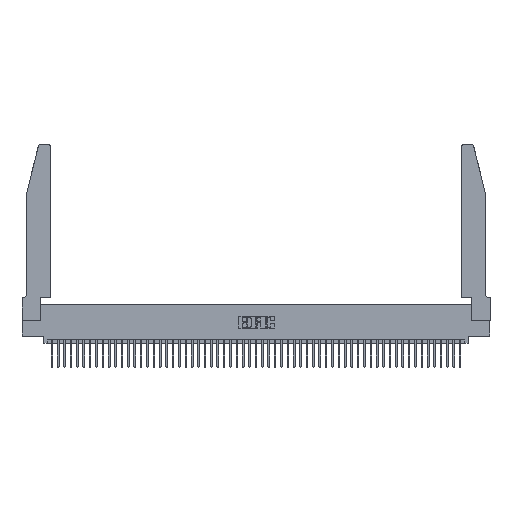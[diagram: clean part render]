
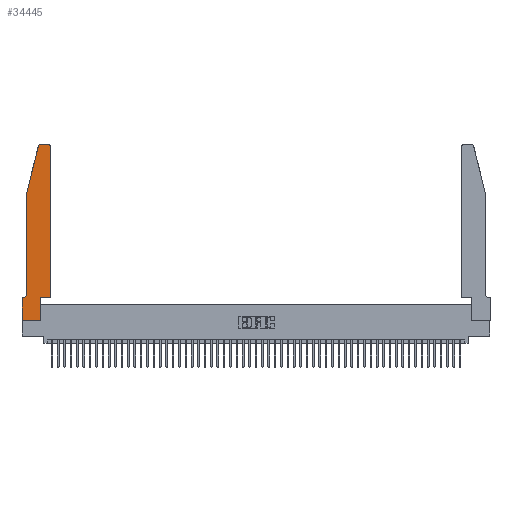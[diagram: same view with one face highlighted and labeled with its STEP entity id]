
A CAD part, top view. The second image highlights one B-rep face of the part: STEP entity #34445.
In plain terms, the highlighted planar face has unit normal (0, 0, 1).
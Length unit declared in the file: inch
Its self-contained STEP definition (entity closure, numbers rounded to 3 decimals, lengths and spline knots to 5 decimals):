
#360 = VERTEX_POINT ( 'NONE', #17462 ) ;
#507 = ORIENTED_EDGE ( 'NONE', *, *, #22948, .T. ) ;
#922 = EDGE_CURVE ( 'NONE', #16100, #12713, #37362, .T. ) ;
#1085 = EDGE_CURVE ( 'NONE', #42099, #38102, #20136, .T. ) ;
#3077 = CARTESIAN_POINT ( 'NONE',  ( 0.284, 2.72, 0.37 ) ) ;
#3145 = CARTESIAN_POINT ( 'NONE',  ( 0.0755, 0.35, 0.37 ) ) ;
#3592 = CARTESIAN_POINT ( 'NONE',  ( 0.0755, 0.42, 0.37 ) ) ;
#3770 = DIRECTION ( 'NONE',  ( 0., 0., -1. ) ) ;
#6470 = EDGE_CURVE ( 'NONE', #20905, #16100, #29015, .T. ) ;
#6724 = LINE ( 'NONE', #24206, #24653 ) ;
#6768 = CARTESIAN_POINT ( 'NONE',  ( 0.284, 2.75, 0.37 ) ) ;
#7198 = DIRECTION ( 'NONE',  ( 1., 0., 0. ) ) ;
#7487 = ORIENTED_EDGE ( 'NONE', *, *, #6470, .T. ) ;
#8018 = DIRECTION ( 'NONE',  ( 0., 1., 0. ) ) ;
#9905 = CIRCLE ( 'NONE', #37328, 0.03 ) ;
#10238 = CARTESIAN_POINT ( 'NONE',  ( 0., 0., 0.37 ) ) ;
#10425 = DIRECTION ( 'NONE',  ( 1., 0., 0. ) ) ;
#10659 = CARTESIAN_POINT ( 'NONE',  ( 0.4205, 2.75, 0.37 ) ) ;
#10813 = CARTESIAN_POINT ( 'NONE',  ( 0.4505, 0.35, 0.37 ) ) ;
#11305 = DIRECTION ( 'NONE',  ( 0., 1., 0. ) ) ;
#11306 = VECTOR ( 'NONE', #48697, 39.37008 ) ;
#11447 = EDGE_CURVE ( 'NONE', #22793, #17503, #43804, .T. ) ;
#12713 = VERTEX_POINT ( 'NONE', #25295 ) ;
#12876 = VERTEX_POINT ( 'NONE', #38445 ) ;
#13257 = VECTOR ( 'NONE', #8018, 39.37008 ) ;
#13656 = ORIENTED_EDGE ( 'NONE', *, *, #922, .T. ) ;
#13734 = VECTOR ( 'NONE', #10425, 39.37008 ) ;
#14359 = CARTESIAN_POINT ( 'NONE',  ( 0.4205, 2.72, 0.37 ) ) ;
#14527 = LINE ( 'NONE', #52760, #13257 ) ;
#14745 = CIRCLE ( 'NONE', #52663, 0.07 ) ;
#14985 = LINE ( 'NONE', #10238, #13734 ) ;
#15666 = VECTOR ( 'NONE', #25620, 39.37008 ) ;
#16100 = VERTEX_POINT ( 'NONE', #22201 ) ;
#16350 = DIRECTION ( 'NONE',  ( 1., 0., 0. ) ) ;
#16436 = VECTOR ( 'NONE', #46405, 39.37008 ) ;
#16897 = DIRECTION ( 'NONE',  ( 0., -1., 0. ) ) ;
#16950 = VECTOR ( 'NONE', #16897, 39.37008 ) ;
#17418 = CARTESIAN_POINT ( 'NONE',  ( 0., 0., 0.37 ) ) ;
#17462 = CARTESIAN_POINT ( 'NONE',  ( 0.0755, 2., 0.37 ) ) ;
#17503 = VERTEX_POINT ( 'NONE', #10813 ) ;
#18164 = VECTOR ( 'NONE', #23723, 39.37008 ) ;
#18384 = VECTOR ( 'NONE', #11305, 39.37008 ) ;
#18457 = DIRECTION ( 'NONE',  ( 1., 0., 0. ) ) ;
#19720 = EDGE_CURVE ( 'NONE', #34900, #22793, #40046, .T. ) ;
#19772 = CARTESIAN_POINT ( 'NONE',  ( 0.2865, 0.35, 0.37 ) ) ;
#20136 = CIRCLE ( 'NONE', #35184, 0.03 ) ;
#20404 = ORIENTED_EDGE ( 'NONE', *, *, #23225, .T. ) ;
#20905 = VERTEX_POINT ( 'NONE', #47005 ) ;
#21064 = EDGE_CURVE ( 'NONE', #28283, #12876, #9905, .T. ) ;
#21547 = EDGE_CURVE ( 'NONE', #52152, #20905, #14745, .T. ) ;
#21848 = EDGE_CURVE ( 'NONE', #12876, #360, #48921, .T. ) ;
#21993 = CARTESIAN_POINT ( 'NONE',  ( 0.0755, 2., 0.37 ) ) ;
#22201 = CARTESIAN_POINT ( 'NONE',  ( 0., 0.35, 0.37 ) ) ;
#22793 = VERTEX_POINT ( 'NONE', #19772 ) ;
#22948 = EDGE_CURVE ( 'NONE', #360, #52152, #27788, .T. ) ;
#23225 = EDGE_CURVE ( 'NONE', #12713, #34900, #14985, .T. ) ;
#23723 = DIRECTION ( 'NONE',  ( -1., 0., 0. ) ) ;
#24206 = CARTESIAN_POINT ( 'NONE',  ( 0.2605, 2.75, 0.37 ) ) ;
#24377 = CARTESIAN_POINT ( 'NONE',  ( 0., 0.35, 0.37 ) ) ;
#24653 = VECTOR ( 'NONE', #40570, 39.37008 ) ;
#25111 = ORIENTED_EDGE ( 'NONE', *, *, #21547, .T. ) ;
#25295 = CARTESIAN_POINT ( 'NONE',  ( 0., 0., 0.37 ) ) ;
#25620 = DIRECTION ( 'NONE',  ( 0., -1., 0. ) ) ;
#26880 = ORIENTED_EDGE ( 'NONE', *, *, #36431, .T. ) ;
#26905 = ORIENTED_EDGE ( 'NONE', *, *, #1085, .T. ) ;
#27788 = LINE ( 'NONE', #37213, #16950 ) ;
#28262 = CARTESIAN_POINT ( 'NONE',  ( 0.0055, 0.42, 0.37 ) ) ;
#28283 = VERTEX_POINT ( 'NONE', #6768 ) ;
#28730 = ORIENTED_EDGE ( 'NONE', *, *, #21064, .T. ) ;
#29015 = LINE ( 'NONE', #3145, #18164 ) ;
#30529 = FACE_OUTER_BOUND ( 'NONE', #33356, .T. ) ;
#31437 = CARTESIAN_POINT ( 'NONE',  ( 0.2865, 0., 0.37 ) ) ;
#31670 = DIRECTION ( 'NONE',  ( 0., 0., 1. ) ) ;
#32353 = DIRECTION ( 'NONE',  ( -1., 0., 0. ) ) ;
#33356 = EDGE_LOOP ( 'NONE', ( #26880, #28730, #48026, #507, #25111, #7487, #13656, #20404, #46982, #50989, #36571, #26905 ) ) ;
#34445 = ADVANCED_FACE ( 'NONE', ( #30529 ), #36675, .T. ) ;
#34900 = VERTEX_POINT ( 'NONE', #31437 ) ;
#35184 = AXIS2_PLACEMENT_3D ( 'NONE', #14359, #42850, #18457 ) ;
#36431 = EDGE_CURVE ( 'NONE', #38102, #28283, #6724, .T. ) ;
#36571 = ORIENTED_EDGE ( 'NONE', *, *, #46801, .T. ) ;
#36675 = PLANE ( 'NONE',  #48913 ) ;
#37028 = CARTESIAN_POINT ( 'NONE',  ( 0.4505, 2.72, 0.37 ) ) ;
#37213 = CARTESIAN_POINT ( 'NONE',  ( 0.0755, 2., 0.37 ) ) ;
#37328 = AXIS2_PLACEMENT_3D ( 'NONE', #3077, #31670, #7198 ) ;
#37362 = LINE ( 'NONE', #17418, #15666 ) ;
#38102 = VERTEX_POINT ( 'NONE', #10659 ) ;
#38445 = CARTESIAN_POINT ( 'NONE',  ( 0.25487, 2.72718, 0.37 ) ) ;
#40046 = LINE ( 'NONE', #43896, #18384 ) ;
#40570 = DIRECTION ( 'NONE',  ( -1., 0., 0. ) ) ;
#40742 = DIRECTION ( 'NONE',  ( 0., 0., 1. ) ) ;
#42099 = VERTEX_POINT ( 'NONE', #37028 ) ;
#42850 = DIRECTION ( 'NONE',  ( 0., 0., 1. ) ) ;
#43804 = LINE ( 'NONE', #44609, #11306 ) ;
#43896 = CARTESIAN_POINT ( 'NONE',  ( 0.2865, 0.35, 0.37 ) ) ;
#44609 = CARTESIAN_POINT ( 'NONE',  ( 0.4505, 0.35, 0.37 ) ) ;
#46405 = DIRECTION ( 'NONE',  ( -0.239, -0.971, 0. ) ) ;
#46801 = EDGE_CURVE ( 'NONE', #17503, #42099, #14527, .T. ) ;
#46982 = ORIENTED_EDGE ( 'NONE', *, *, #19720, .T. ) ;
#47005 = CARTESIAN_POINT ( 'NONE',  ( 0.0055, 0.35, 0.37 ) ) ;
#48026 = ORIENTED_EDGE ( 'NONE', *, *, #21848, .T. ) ;
#48697 = DIRECTION ( 'NONE',  ( 1., 0., 0. ) ) ;
#48913 = AXIS2_PLACEMENT_3D ( 'NONE', #24377, #40742, #16350 ) ;
#48921 = LINE ( 'NONE', #21993, #16436 ) ;
#50989 = ORIENTED_EDGE ( 'NONE', *, *, #11447, .T. ) ;
#52152 = VERTEX_POINT ( 'NONE', #3592 ) ;
#52663 = AXIS2_PLACEMENT_3D ( 'NONE', #28262, #3770, #32353 ) ;
#52760 = CARTESIAN_POINT ( 'NONE',  ( 0.4505, 0.35, 0.37 ) ) ;
